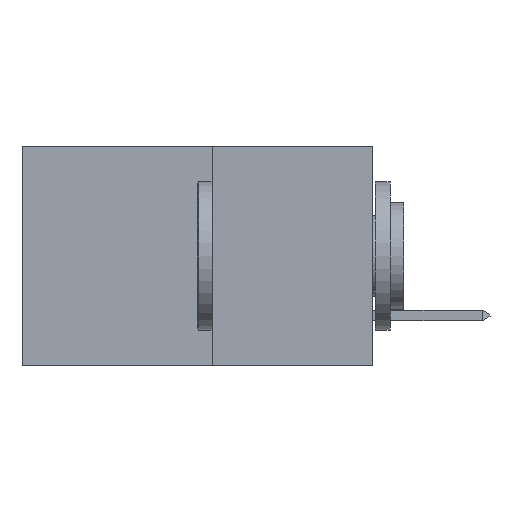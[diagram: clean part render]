
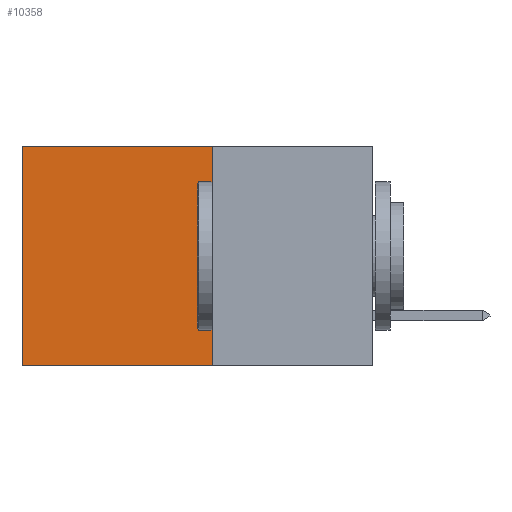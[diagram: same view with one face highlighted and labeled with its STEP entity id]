
A CAD part, left-side view. The second image highlights one B-rep face of the part: STEP entity #10358.
In plain terms, the highlighted planar face has unit normal (-1, 0, 0).
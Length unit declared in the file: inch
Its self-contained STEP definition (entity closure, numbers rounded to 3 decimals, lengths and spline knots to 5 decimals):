
#167 = DIRECTION ( 'NONE',  ( 0., 0., -1. ) ) ;
#195 = DIRECTION ( 'NONE',  ( 0., 1., 0. ) ) ;
#689 = ORIENTED_EDGE ( 'NONE', *, *, #5113, .T. ) ;
#1471 = EDGE_CURVE ( 'NONE', #4734, #2923, #9133, .T. ) ;
#2199 = CARTESIAN_POINT ( 'NONE',  ( 0.277, 0.27, -0.37 ) ) ;
#2679 = DIRECTION ( 'NONE',  ( 0., 1., 0. ) ) ;
#2923 = VERTEX_POINT ( 'NONE', #7438 ) ;
#2991 = LINE ( 'NONE', #8782, #7228 ) ;
#3003 = ORIENTED_EDGE ( 'NONE', *, *, #8749, .F. ) ;
#3079 = AXIS2_PLACEMENT_3D ( 'NONE', #10114, #5377, #167 ) ;
#3098 = LINE ( 'NONE', #5413, #7570 ) ;
#3533 = ORIENTED_EDGE ( 'NONE', *, *, #1471, .T. ) ;
#3972 = VERTEX_POINT ( 'NONE', #10175 ) ;
#4174 = VERTEX_POINT ( 'NONE', #5248 ) ;
#4703 = FACE_OUTER_BOUND ( 'NONE', #6899, .T. ) ;
#4734 = VERTEX_POINT ( 'NONE', #7928 ) ;
#4832 = VECTOR ( 'NONE', #2679, 39.37008 ) ;
#5113 = EDGE_CURVE ( 'NONE', #2923, #3972, #2991, .T. ) ;
#5248 = CARTESIAN_POINT ( 'NONE',  ( 0.277, 0.27, -0.37 ) ) ;
#5290 = ORIENTED_EDGE ( 'NONE', *, *, #9479, .F. ) ;
#5377 = DIRECTION ( 'NONE',  ( 1., 0., 0. ) ) ;
#5413 = CARTESIAN_POINT ( 'NONE',  ( 0.277, 0.27, -0.37 ) ) ;
#6744 = CARTESIAN_POINT ( 'NONE',  ( 0.277, 0.27, 0. ) ) ;
#6899 = EDGE_LOOP ( 'NONE', ( #689, #3003, #5290, #3533 ) ) ;
#7002 = PLANE ( 'NONE',  #3079 ) ;
#7228 = VECTOR ( 'NONE', #8868, 39.37008 ) ;
#7438 = CARTESIAN_POINT ( 'NONE',  ( 0.277, 0.59, 0. ) ) ;
#7570 = VECTOR ( 'NONE', #195, 39.37008 ) ;
#7928 = CARTESIAN_POINT ( 'NONE',  ( 0.277, 0.27, 0. ) ) ;
#8210 = LINE ( 'NONE', #2199, #9983 ) ;
#8749 = EDGE_CURVE ( 'NONE', #4174, #3972, #3098, .T. ) ;
#8782 = CARTESIAN_POINT ( 'NONE',  ( 0.277, 0.59, -0.37 ) ) ;
#8832 = DIRECTION ( 'NONE',  ( 0., 0., -1. ) ) ;
#8868 = DIRECTION ( 'NONE',  ( 0., 0., -1. ) ) ;
#9133 = LINE ( 'NONE', #6744, #4832 ) ;
#9479 = EDGE_CURVE ( 'NONE', #4734, #4174, #8210, .T. ) ;
#9983 = VECTOR ( 'NONE', #8832, 39.37008 ) ;
#10114 = CARTESIAN_POINT ( 'NONE',  ( 0.277, 0.27, -0.37 ) ) ;
#10175 = CARTESIAN_POINT ( 'NONE',  ( 0.277, 0.59, -0.37 ) ) ;
#10358 = ADVANCED_FACE ( 'NONE', ( #4703 ), #7002, .F. ) ;
